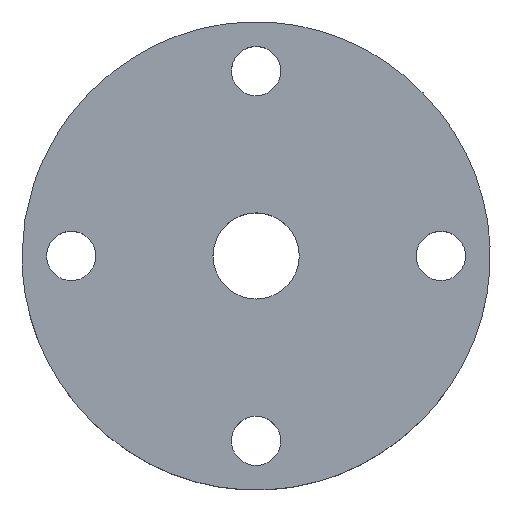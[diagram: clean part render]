
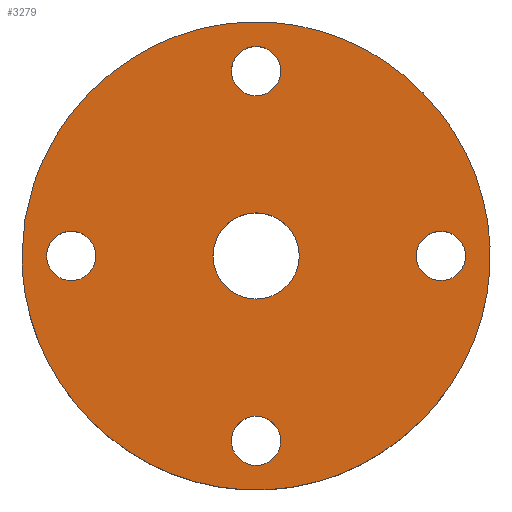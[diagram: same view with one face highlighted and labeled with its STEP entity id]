
A CAD part, top view. The second image highlights one B-rep face of the part: STEP entity #3279.
In plain terms, the highlighted planar face has unit normal (0, 0, 1).
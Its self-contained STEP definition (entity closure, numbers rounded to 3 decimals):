
#26=CIRCLE('',#3352,2.);
#27=CIRCLE('',#3354,2.);
#28=CIRCLE('',#3356,2.);
#29=CIRCLE('',#3358,2.);
#30=CIRCLE('',#3360,3.5);
#32=(
BOUNDED_CURVE()
B_SPLINE_CURVE(5,(#6749,#6750,#6751,#6752,#6753,#6754,#6755,#6756,#6757,
#6758,#6759,#6760,#6761,#6762,#6763,#6764,#6765,#6766,#6767,#6768,#6769,
#6770,#6771,#6772,#6773),.UNSPECIFIED.,.T.,.F.)
B_SPLINE_CURVE_WITH_KNOTS((6,1,1,1,1,1,1,1,1,1,1,1,1,1,1,1,1,1,1,1,6),(0.,
0.05,0.1,0.15,0.2,0.25,0.3,0.35,0.4,0.45,0.5,0.55,0.6,0.65,0.7,0.75,0.8,
0.85,0.9,0.95,1.),.UNSPECIFIED.)
CURVE()
GEOMETRIC_REPRESENTATION_ITEM()
RATIONAL_B_SPLINE_CURVE((1.,1.,1.,1.,1.,1.,1.,1.,1.,1.,1.,1.,1.,1.,1.,1.,
1.,1.,1.,1.,1.,1.,1.,1.,1.))
REPRESENTATION_ITEM('')
);
#47=FACE_BOUND('',#756,.T.);
#48=FACE_BOUND('',#757,.T.);
#49=FACE_BOUND('',#758,.T.);
#50=FACE_BOUND('',#759,.T.);
#51=FACE_BOUND('',#760,.T.);
#567=FACE_OUTER_BOUND('',#755,.T.);
#755=EDGE_LOOP('',(#3046));
#756=EDGE_LOOP('',(#3047));
#757=EDGE_LOOP('',(#3048));
#758=EDGE_LOOP('',(#3049));
#759=EDGE_LOOP('',(#3050));
#760=EDGE_LOOP('',(#3051));
#1579=VERTEX_POINT('',#6679);
#1580=VERTEX_POINT('',#6683);
#1581=VERTEX_POINT('',#6687);
#1582=VERTEX_POINT('',#6691);
#1583=VERTEX_POINT('',#6695);
#1584=VERTEX_POINT('',#6748);
#2063=EDGE_CURVE('',#1579,#1579,#26,.T.);
#2065=EDGE_CURVE('',#1580,#1580,#27,.T.);
#2067=EDGE_CURVE('',#1581,#1581,#28,.T.);
#2069=EDGE_CURVE('',#1582,#1582,#29,.T.);
#2071=EDGE_CURVE('',#1583,#1583,#30,.T.);
#2072=EDGE_CURVE('',#1584,#1584,#32,.T.);
#3046=ORIENTED_EDGE('',*,*,#2072,.F.);
#3047=ORIENTED_EDGE('',*,*,#2071,.F.);
#3048=ORIENTED_EDGE('',*,*,#2069,.F.);
#3049=ORIENTED_EDGE('',*,*,#2067,.F.);
#3050=ORIENTED_EDGE('',*,*,#2065,.F.);
#3051=ORIENTED_EDGE('',*,*,#2063,.F.);
#3105=PLANE('',#3362);
#3279=ADVANCED_FACE('',(#567,#47,#48,#49,#50,#51),#3105,.F.);
#3352=AXIS2_PLACEMENT_3D('',#6681,#3725,#3726);
#3354=AXIS2_PLACEMENT_3D('',#6685,#3730,#3731);
#3356=AXIS2_PLACEMENT_3D('',#6689,#3735,#3736);
#3358=AXIS2_PLACEMENT_3D('',#6693,#3740,#3741);
#3360=AXIS2_PLACEMENT_3D('',#6697,#3745,#3746);
#3362=AXIS2_PLACEMENT_3D('',#6776,#3750,#3751);
#3725=DIRECTION('center_axis',(0.,0.,1.));
#3726=DIRECTION('ref_axis',(1.,0.,0.));
#3730=DIRECTION('center_axis',(0.,0.,1.));
#3731=DIRECTION('ref_axis',(1.,0.,0.));
#3735=DIRECTION('center_axis',(0.,0.,1.));
#3736=DIRECTION('ref_axis',(1.,0.,0.));
#3740=DIRECTION('center_axis',(0.,0.,1.));
#3741=DIRECTION('ref_axis',(1.,0.,0.));
#3745=DIRECTION('center_axis',(0.,0.,1.));
#3746=DIRECTION('ref_axis',(1.,0.,0.));
#3750=DIRECTION('center_axis',(0.,0.,-1.));
#3751=DIRECTION('ref_axis',(1.,0.,0.));
#6679=CARTESIAN_POINT('',(48.,20.,0.));
#6681=CARTESIAN_POINT('Origin',(50.,20.,0.));
#6683=CARTESIAN_POINT('',(18.,20.,0.));
#6685=CARTESIAN_POINT('Origin',(20.,20.,0.));
#6687=CARTESIAN_POINT('',(33.,35.,0.));
#6689=CARTESIAN_POINT('Origin',(35.,35.,0.));
#6691=CARTESIAN_POINT('',(33.,5.,0.));
#6693=CARTESIAN_POINT('Origin',(35.,5.,0.));
#6695=CARTESIAN_POINT('',(31.5,20.,0.));
#6697=CARTESIAN_POINT('Origin',(35.,20.,0.));
#6748=CARTESIAN_POINT('',(16.,20.,0.));
#6749=CARTESIAN_POINT('Ctrl Pts',(16.,20.,0.));
#6750=CARTESIAN_POINT('Ctrl Pts',(16.,21.186,0.));
#6751=CARTESIAN_POINT('Ctrl Pts',(16.19,23.559,0.));
#6752=CARTESIAN_POINT('Ctrl Pts',(17.048,27.061,0.));
#6753=CARTESIAN_POINT('Ctrl Pts',(19.286,31.391,0.));
#6754=CARTESIAN_POINT('Ctrl Pts',(23.609,35.714,0.));
#6755=CARTESIAN_POINT('Ctrl Pts',(29.021,38.512,0.));
#6756=CARTESIAN_POINT('Ctrl Pts',(35.,39.484,0.));
#6757=CARTESIAN_POINT('Ctrl Pts',(40.979,38.512,0.));
#6758=CARTESIAN_POINT('Ctrl Pts',(46.391,35.714,0.));
#6759=CARTESIAN_POINT('Ctrl Pts',(50.714,31.391,0.));
#6760=CARTESIAN_POINT('Ctrl Pts',(53.512,25.979,0.));
#6761=CARTESIAN_POINT('Ctrl Pts',(54.484,20.,0.));
#6762=CARTESIAN_POINT('Ctrl Pts',(53.512,14.021,0.));
#6763=CARTESIAN_POINT('Ctrl Pts',(50.714,8.609,0.));
#6764=CARTESIAN_POINT('Ctrl Pts',(46.391,4.286,0.));
#6765=CARTESIAN_POINT('Ctrl Pts',(40.979,1.488,0.));
#6766=CARTESIAN_POINT('Ctrl Pts',(35.,0.516,0.));
#6767=CARTESIAN_POINT('Ctrl Pts',(29.021,1.488,0.));
#6768=CARTESIAN_POINT('Ctrl Pts',(23.609,4.286,0.));
#6769=CARTESIAN_POINT('Ctrl Pts',(19.286,8.609,0.));
#6770=CARTESIAN_POINT('Ctrl Pts',(17.048,12.939,0.));
#6771=CARTESIAN_POINT('Ctrl Pts',(16.19,16.441,0.));
#6772=CARTESIAN_POINT('Ctrl Pts',(16.,18.814,0.));
#6773=CARTESIAN_POINT('Ctrl Pts',(16.,20.,0.));
#6776=CARTESIAN_POINT('Origin',(35.242,20.,0.));
